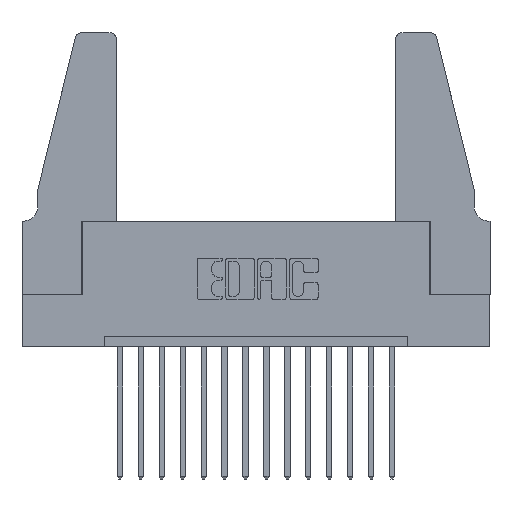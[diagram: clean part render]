
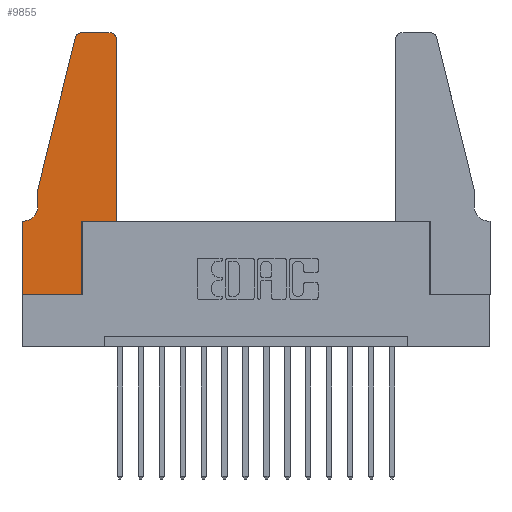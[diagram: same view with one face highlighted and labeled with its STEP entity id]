
A CAD part, top view. The second image highlights one B-rep face of the part: STEP entity #9855.
In plain terms, the highlighted planar face has unit normal (0, 0, 1).
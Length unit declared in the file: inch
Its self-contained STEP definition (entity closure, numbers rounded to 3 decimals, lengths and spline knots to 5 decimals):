
#281 = EDGE_LOOP ( 'NONE', ( #589, #8311, #8930, #7379, #4612, #2898, #15370, #6576, #1523, #8050, #5834, #7663 ) ) ;
#354 = LINE ( 'NONE', #14808, #2108 ) ;
#557 = CARTESIAN_POINT ( 'NONE',  ( 0.2865, 0.35, 0.37 ) ) ;
#589 = ORIENTED_EDGE ( 'NONE', *, *, #7466, .T. ) ;
#1491 = CARTESIAN_POINT ( 'NONE',  ( 0.4505, 0.35, 0.37 ) ) ;
#1523 = ORIENTED_EDGE ( 'NONE', *, *, #2144, .T. ) ;
#1687 = VECTOR ( 'NONE', #5885, 39.37008 ) ;
#1793 = VERTEX_POINT ( 'NONE', #13916 ) ;
#1795 = CARTESIAN_POINT ( 'NONE',  ( 0., 0.35, 0.37 ) ) ;
#1798 = CARTESIAN_POINT ( 'NONE',  ( 0.0755, 0.35, 0.37 ) ) ;
#1994 = LINE ( 'NONE', #9435, #16393 ) ;
#2108 = VECTOR ( 'NONE', #10921, 39.37008 ) ;
#2144 = EDGE_CURVE ( 'NONE', #7029, #16465, #5068, .T. ) ;
#2508 = AXIS2_PLACEMENT_3D ( 'NONE', #9802, #6157, #3443 ) ;
#2519 = CARTESIAN_POINT ( 'NONE',  ( 0.4505, 1.22, 0.37 ) ) ;
#2563 = EDGE_CURVE ( 'NONE', #10398, #4935, #7848, .T. ) ;
#2607 = CARTESIAN_POINT ( 'NONE',  ( 0., 0., 0.37 ) ) ;
#2811 = DIRECTION ( 'NONE',  ( 1., 0., 0. ) ) ;
#2866 = DIRECTION ( 'NONE',  ( 0., 0., 1. ) ) ;
#2898 = ORIENTED_EDGE ( 'NONE', *, *, #16192, .T. ) ;
#3132 = VERTEX_POINT ( 'NONE', #2607 ) ;
#3443 = DIRECTION ( 'NONE',  ( 1., 0., 0. ) ) ;
#4010 = DIRECTION ( 'NONE',  ( -1., 0., 0. ) ) ;
#4408 = CIRCLE ( 'NONE', #7459, 0.03 ) ;
#4612 = ORIENTED_EDGE ( 'NONE', *, *, #11083, .T. ) ;
#4935 = VERTEX_POINT ( 'NONE', #15106 ) ;
#4936 = CARTESIAN_POINT ( 'NONE',  ( 0.25487, 1.22718, 0.37 ) ) ;
#5068 = LINE ( 'NONE', #10884, #1687 ) ;
#5434 = EDGE_CURVE ( 'NONE', #10619, #6763, #13743, .T. ) ;
#5472 = CIRCLE ( 'NONE', #10628, 0.07 ) ;
#5645 = EDGE_CURVE ( 'NONE', #4935, #15013, #11218, .T. ) ;
#5834 = ORIENTED_EDGE ( 'NONE', *, *, #5434, .T. ) ;
#5885 = DIRECTION ( 'NONE',  ( 0., 1., 0. ) ) ;
#6056 = DIRECTION ( 'NONE',  ( 1., 0., 0. ) ) ;
#6157 = DIRECTION ( 'NONE',  ( 0., 0., 1. ) ) ;
#6434 = CARTESIAN_POINT ( 'NONE',  ( 0.284, 1.25, 0.37 ) ) ;
#6576 = ORIENTED_EDGE ( 'NONE', *, *, #13703, .T. ) ;
#6750 = PLANE ( 'NONE',  #9025 ) ;
#6763 = VERTEX_POINT ( 'NONE', #2519 ) ;
#6788 = VECTOR ( 'NONE', #12237, 39.37008 ) ;
#6872 = DIRECTION ( 'NONE',  ( 1., 0., 0. ) ) ;
#6908 = DIRECTION ( 'NONE',  ( -1., 0., 0. ) ) ;
#6911 = VECTOR ( 'NONE', #6908, 39.37008 ) ;
#6954 = VECTOR ( 'NONE', #7342, 39.37008 ) ;
#7029 = VERTEX_POINT ( 'NONE', #15631 ) ;
#7342 = DIRECTION ( 'NONE',  ( 0., 1., 0. ) ) ;
#7379 = ORIENTED_EDGE ( 'NONE', *, *, #5645, .T. ) ;
#7459 = AXIS2_PLACEMENT_3D ( 'NONE', #9975, #15042, #6056 ) ;
#7466 = EDGE_CURVE ( 'NONE', #11030, #7964, #8803, .T. ) ;
#7521 = CIRCLE ( 'NONE', #2508, 0.03 ) ;
#7663 = ORIENTED_EDGE ( 'NONE', *, *, #12994, .T. ) ;
#7848 = LINE ( 'NONE', #15491, #13826 ) ;
#7964 = VERTEX_POINT ( 'NONE', #6434 ) ;
#8050 = ORIENTED_EDGE ( 'NONE', *, *, #9966, .T. ) ;
#8311 = ORIENTED_EDGE ( 'NONE', *, *, #15900, .T. ) ;
#8803 = LINE ( 'NONE', #13019, #10414 ) ;
#8930 = ORIENTED_EDGE ( 'NONE', *, *, #2563, .T. ) ;
#9025 = AXIS2_PLACEMENT_3D ( 'NONE', #13118, #2866, #2811 ) ;
#9148 = DIRECTION ( 'NONE',  ( -0.239, -0.971, 0. ) ) ;
#9212 = DIRECTION ( 'NONE',  ( 0., -1., 0. ) ) ;
#9391 = CARTESIAN_POINT ( 'NONE',  ( 0.0755, 0.42, 0.37 ) ) ;
#9435 = CARTESIAN_POINT ( 'NONE',  ( 0., 0., 0.37 ) ) ;
#9711 = LINE ( 'NONE', #1798, #6911 ) ;
#9739 = CARTESIAN_POINT ( 'NONE',  ( 0.4505, 0.35, 0.37 ) ) ;
#9802 = CARTESIAN_POINT ( 'NONE',  ( 0.284, 1.22, 0.37 ) ) ;
#9855 = ADVANCED_FACE ( 'NONE', ( #11935 ), #6750, .T. ) ;
#9966 = EDGE_CURVE ( 'NONE', #16465, #10619, #354, .T. ) ;
#9975 = CARTESIAN_POINT ( 'NONE',  ( 0.4205, 1.22, 0.37 ) ) ;
#10159 = DIRECTION ( 'NONE',  ( 0., 0., -1. ) ) ;
#10398 = VERTEX_POINT ( 'NONE', #4936 ) ;
#10414 = VECTOR ( 'NONE', #4010, 39.37008 ) ;
#10619 = VERTEX_POINT ( 'NONE', #1491 ) ;
#10628 = AXIS2_PLACEMENT_3D ( 'NONE', #13907, #10159, #15103 ) ;
#10884 = CARTESIAN_POINT ( 'NONE',  ( 0.2865, 0.35, 0.37 ) ) ;
#10921 = DIRECTION ( 'NONE',  ( 1., 0., 0. ) ) ;
#10954 = CARTESIAN_POINT ( 'NONE',  ( 0.0755, 0.5, 0.37 ) ) ;
#11030 = VERTEX_POINT ( 'NONE', #14331 ) ;
#11083 = EDGE_CURVE ( 'NONE', #15013, #1793, #5472, .T. ) ;
#11218 = LINE ( 'NONE', #10954, #6788 ) ;
#11901 = VERTEX_POINT ( 'NONE', #1795 ) ;
#11935 = FACE_OUTER_BOUND ( 'NONE', #281, .T. ) ;
#12237 = DIRECTION ( 'NONE',  ( 0., -1., 0. ) ) ;
#12599 = EDGE_CURVE ( 'NONE', #11901, #3132, #15632, .T. ) ;
#12994 = EDGE_CURVE ( 'NONE', #6763, #11030, #4408, .T. ) ;
#13019 = CARTESIAN_POINT ( 'NONE',  ( 0.2605, 1.25, 0.37 ) ) ;
#13118 = CARTESIAN_POINT ( 'NONE',  ( 0., 0.35, 0.37 ) ) ;
#13461 = VECTOR ( 'NONE', #9212, 39.37008 ) ;
#13703 = EDGE_CURVE ( 'NONE', #3132, #7029, #1994, .T. ) ;
#13743 = LINE ( 'NONE', #9739, #6954 ) ;
#13826 = VECTOR ( 'NONE', #9148, 39.37008 ) ;
#13907 = CARTESIAN_POINT ( 'NONE',  ( 0.0055, 0.42, 0.37 ) ) ;
#13916 = CARTESIAN_POINT ( 'NONE',  ( 0.0055, 0.35, 0.37 ) ) ;
#14331 = CARTESIAN_POINT ( 'NONE',  ( 0.4205, 1.25, 0.37 ) ) ;
#14808 = CARTESIAN_POINT ( 'NONE',  ( 0.4505, 0.35, 0.37 ) ) ;
#15013 = VERTEX_POINT ( 'NONE', #9391 ) ;
#15042 = DIRECTION ( 'NONE',  ( 0., 0., 1. ) ) ;
#15103 = DIRECTION ( 'NONE',  ( -1., 0., 0. ) ) ;
#15106 = CARTESIAN_POINT ( 'NONE',  ( 0.0755, 0.5, 0.37 ) ) ;
#15370 = ORIENTED_EDGE ( 'NONE', *, *, #12599, .T. ) ;
#15491 = CARTESIAN_POINT ( 'NONE',  ( 0.0755, 0.5, 0.37 ) ) ;
#15561 = CARTESIAN_POINT ( 'NONE',  ( 0., 0., 0.37 ) ) ;
#15631 = CARTESIAN_POINT ( 'NONE',  ( 0.2865, 0., 0.37 ) ) ;
#15632 = LINE ( 'NONE', #15561, #13461 ) ;
#15900 = EDGE_CURVE ( 'NONE', #7964, #10398, #7521, .T. ) ;
#16192 = EDGE_CURVE ( 'NONE', #1793, #11901, #9711, .T. ) ;
#16393 = VECTOR ( 'NONE', #6872, 39.37008 ) ;
#16465 = VERTEX_POINT ( 'NONE', #557 ) ;
